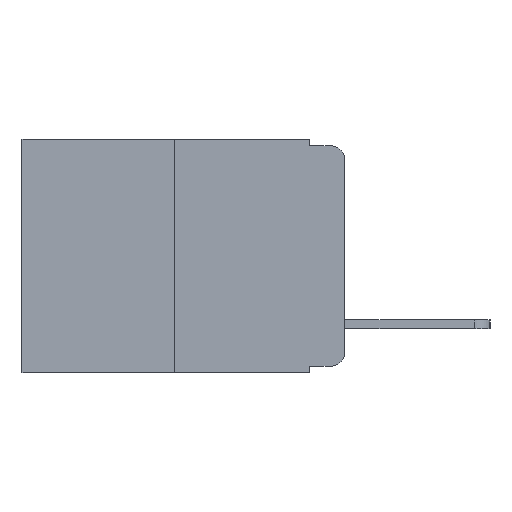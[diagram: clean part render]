
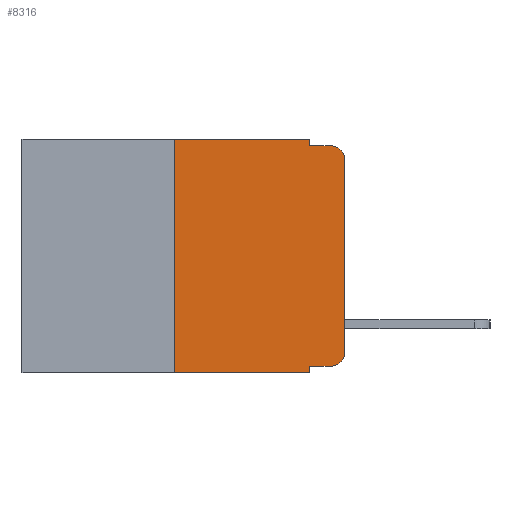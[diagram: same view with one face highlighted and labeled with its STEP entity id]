
A CAD part, left-side view. The second image highlights one B-rep face of the part: STEP entity #8316.
In plain terms, the highlighted planar face has unit normal (-1, 0, 0).
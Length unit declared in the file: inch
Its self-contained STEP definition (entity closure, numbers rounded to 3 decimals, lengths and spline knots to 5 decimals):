
#217 = FACE_OUTER_BOUND ( 'NONE', #12979, .T. ) ;
#548 = LINE ( 'NONE', #12320, #14600 ) ;
#781 = CARTESIAN_POINT ( 'NONE',  ( 0., 0.473, 0. ) ) ;
#890 = CARTESIAN_POINT ( 'NONE',  ( 0., 0.473, -0.343 ) ) ;
#964 = AXIS2_PLACEMENT_3D ( 'NONE', #16932, #9955, #1254 ) ;
#1206 = DIRECTION ( 'NONE',  ( 0., -1., 0. ) ) ;
#1254 = DIRECTION ( 'NONE',  ( 0., 0., -1. ) ) ;
#2403 = PLANE ( 'NONE',  #7134 ) ;
#2424 = LINE ( 'NONE', #11042, #12928 ) ;
#2781 = VERTEX_POINT ( 'NONE', #3676 ) ;
#3447 = CARTESIAN_POINT ( 'NONE',  ( 0., 0., -0.313 ) ) ;
#3676 = CARTESIAN_POINT ( 'NONE',  ( 0., 0.02, -0.01 ) ) ;
#3956 = DIRECTION ( 'NONE',  ( 0., -1., 0. ) ) ;
#4657 = CARTESIAN_POINT ( 'NONE',  ( 0., 0.051, -0.343 ) ) ;
#4780 = VECTOR ( 'NONE', #5577, 39.37008 ) ;
#4927 = EDGE_CURVE ( 'NONE', #13233, #17049, #548, .T. ) ;
#4947 = VERTEX_POINT ( 'NONE', #7256 ) ;
#5081 = VERTEX_POINT ( 'NONE', #12383 ) ;
#5203 = DIRECTION ( 'NONE',  ( 0., 0., -1. ) ) ;
#5245 = CIRCLE ( 'NONE', #964, 0.02 ) ;
#5276 = VECTOR ( 'NONE', #9790, 39.37008 ) ;
#5577 = DIRECTION ( 'NONE',  ( 0., 0., 1. ) ) ;
#6195 = VECTOR ( 'NONE', #12484, 39.37008 ) ;
#6262 = EDGE_CURVE ( 'NONE', #9667, #12905, #8095, .T. ) ;
#6356 = CARTESIAN_POINT ( 'NONE',  ( 0., 0.051, -0.01 ) ) ;
#6634 = LINE ( 'NONE', #13456, #13299 ) ;
#6854 = DIRECTION ( 'NONE',  ( 0., 0., -1. ) ) ;
#7134 = AXIS2_PLACEMENT_3D ( 'NONE', #781, #13302, #5203 ) ;
#7201 = CARTESIAN_POINT ( 'NONE',  ( 0., 0.02, -0.313 ) ) ;
#7256 = CARTESIAN_POINT ( 'NONE',  ( 0., 0., -0.03 ) ) ;
#7281 = VERTEX_POINT ( 'NONE', #6356 ) ;
#7766 = EDGE_CURVE ( 'NONE', #9667, #13233, #15623, .T. ) ;
#7969 = VERTEX_POINT ( 'NONE', #3447 ) ;
#7981 = EDGE_CURVE ( 'NONE', #17049, #7281, #8066, .T. ) ;
#8026 = EDGE_CURVE ( 'NONE', #7281, #2781, #16317, .T. ) ;
#8049 = EDGE_CURVE ( 'NONE', #12378, #7969, #12943, .T. ) ;
#8066 = LINE ( 'NONE', #14623, #14401 ) ;
#8095 = LINE ( 'NONE', #890, #14766 ) ;
#8149 = DIRECTION ( 'NONE',  ( 0., -1., 0. ) ) ;
#8303 = CARTESIAN_POINT ( 'NONE',  ( 0., 0.25, 0. ) ) ;
#8316 = ADVANCED_FACE ( 'NONE', ( #217 ), #2403, .F. ) ;
#8395 = EDGE_CURVE ( 'NONE', #5081, #12378, #6634, .T. ) ;
#8399 = EDGE_CURVE ( 'NONE', #5081, #12905, #2424, .T. ) ;
#8423 = EDGE_CURVE ( 'NONE', #4947, #2781, #5245, .T. ) ;
#8444 = EDGE_CURVE ( 'NONE', #7969, #4947, #8694, .T. ) ;
#8675 = DIRECTION ( 'NONE',  ( 0., 0., -1. ) ) ;
#8694 = LINE ( 'NONE', #10015, #4780 ) ;
#9055 = CARTESIAN_POINT ( 'NONE',  ( 0., 0.051, 0. ) ) ;
#9667 = VERTEX_POINT ( 'NONE', #16051 ) ;
#9790 = DIRECTION ( 'NONE',  ( 0., 0., 1. ) ) ;
#9955 = DIRECTION ( 'NONE',  ( -1., 0., 0. ) ) ;
#10015 = CARTESIAN_POINT ( 'NONE',  ( 0., 0., 0. ) ) ;
#11042 = CARTESIAN_POINT ( 'NONE',  ( 0., 0.051, 0. ) ) ;
#11093 = ORIENTED_EDGE ( 'NONE', *, *, #8444, .T. ) ;
#11108 = ORIENTED_EDGE ( 'NONE', *, *, #8423, .T. ) ;
#11269 = CARTESIAN_POINT ( 'NONE',  ( 0., 0.051, -0.01 ) ) ;
#11430 = ORIENTED_EDGE ( 'NONE', *, *, #8026, .F. ) ;
#11441 = ORIENTED_EDGE ( 'NONE', *, *, #7981, .F. ) ;
#11979 = ORIENTED_EDGE ( 'NONE', *, *, #4927, .F. ) ;
#12073 = CARTESIAN_POINT ( 'NONE',  ( 0., 0.25, 0. ) ) ;
#12170 = ORIENTED_EDGE ( 'NONE', *, *, #7766, .F. ) ;
#12172 = ORIENTED_EDGE ( 'NONE', *, *, #6262, .T. ) ;
#12320 = CARTESIAN_POINT ( 'NONE',  ( 0., 0.473, 0. ) ) ;
#12378 = VERTEX_POINT ( 'NONE', #14734 ) ;
#12383 = CARTESIAN_POINT ( 'NONE',  ( 0., 0.051, -0.333 ) ) ;
#12426 = ORIENTED_EDGE ( 'NONE', *, *, #8399, .F. ) ;
#12484 = DIRECTION ( 'NONE',  ( 0., -1., 0. ) ) ;
#12549 = ORIENTED_EDGE ( 'NONE', *, *, #8395, .T. ) ;
#12583 = ORIENTED_EDGE ( 'NONE', *, *, #8049, .T. ) ;
#12905 = VERTEX_POINT ( 'NONE', #4657 ) ;
#12928 = VECTOR ( 'NONE', #6854, 39.37008 ) ;
#12943 = CIRCLE ( 'NONE', #13434, 0.02 ) ;
#12979 = EDGE_LOOP ( 'NONE', ( #11093, #11108, #11430, #11441, #11979, #12170, #12172, #12426, #12549, #12583 ) ) ;
#13233 = VERTEX_POINT ( 'NONE', #12073 ) ;
#13299 = VECTOR ( 'NONE', #3956, 39.37008 ) ;
#13302 = DIRECTION ( 'NONE',  ( 1., 0., 0. ) ) ;
#13434 = AXIS2_PLACEMENT_3D ( 'NONE', #7201, #15977, #8675 ) ;
#13456 = CARTESIAN_POINT ( 'NONE',  ( 0., 0.051, -0.333 ) ) ;
#14401 = VECTOR ( 'NONE', #15744, 39.37008 ) ;
#14600 = VECTOR ( 'NONE', #1206, 39.37008 ) ;
#14623 = CARTESIAN_POINT ( 'NONE',  ( 0., 0.051, 0. ) ) ;
#14734 = CARTESIAN_POINT ( 'NONE',  ( 0., 0.02, -0.333 ) ) ;
#14766 = VECTOR ( 'NONE', #8149, 39.37008 ) ;
#15623 = LINE ( 'NONE', #8303, #5276 ) ;
#15744 = DIRECTION ( 'NONE',  ( 0., 0., -1. ) ) ;
#15977 = DIRECTION ( 'NONE',  ( -1., 0., 0. ) ) ;
#16051 = CARTESIAN_POINT ( 'NONE',  ( 0., 0.25, -0.343 ) ) ;
#16317 = LINE ( 'NONE', #11269, #6195 ) ;
#16932 = CARTESIAN_POINT ( 'NONE',  ( 0., 0.02, -0.03 ) ) ;
#17049 = VERTEX_POINT ( 'NONE', #9055 ) ;
